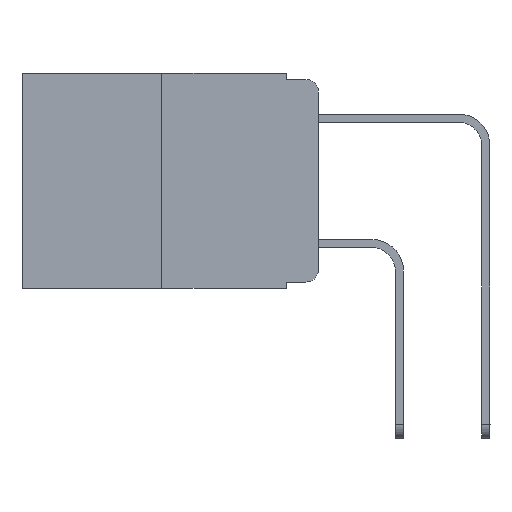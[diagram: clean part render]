
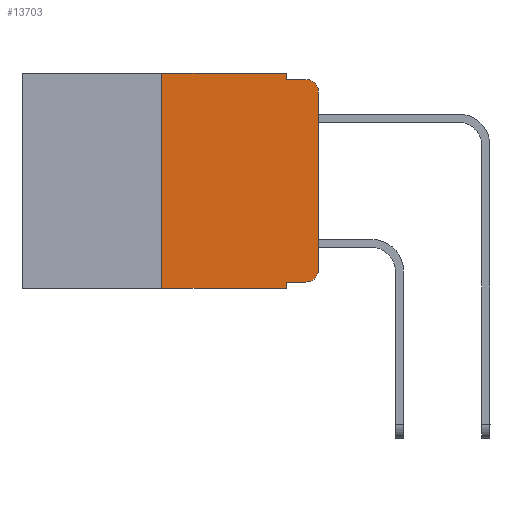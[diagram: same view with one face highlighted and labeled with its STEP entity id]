
A CAD part, left-side view. The second image highlights one B-rep face of the part: STEP entity #13703.
In plain terms, the highlighted planar face has unit normal (-1, 0, 0).
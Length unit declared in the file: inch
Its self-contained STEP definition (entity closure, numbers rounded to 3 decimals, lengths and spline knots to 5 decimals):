
#487 = DIRECTION ( 'NONE',  ( 0., -1., 0. ) ) ;
#741 = EDGE_CURVE ( 'NONE', #13259, #19435, #17257, .T. ) ;
#805 = DIRECTION ( 'NONE',  ( 0., -1., 0. ) ) ;
#1256 = CARTESIAN_POINT ( 'NONE',  ( 0., 0.02, -0.333 ) ) ;
#1263 = VERTEX_POINT ( 'NONE', #3067 ) ;
#1503 = LINE ( 'NONE', #21283, #15913 ) ;
#2000 = EDGE_CURVE ( 'NONE', #12940, #22669, #3964, .T. ) ;
#2510 = LINE ( 'NONE', #9604, #2660 ) ;
#2660 = VECTOR ( 'NONE', #16778, 39.37008 ) ;
#3067 = CARTESIAN_POINT ( 'NONE',  ( 0., 0.051, -0.333 ) ) ;
#3137 = LINE ( 'NONE', #13869, #8609 ) ;
#3624 = DIRECTION ( 'NONE',  ( 0., -1., 0. ) ) ;
#3964 = LINE ( 'NONE', #22002, #16583 ) ;
#4494 = VERTEX_POINT ( 'NONE', #10159 ) ;
#4611 = DIRECTION ( 'NONE',  ( 0., 0., 1. ) ) ;
#4775 = ORIENTED_EDGE ( 'NONE', *, *, #2000, .F. ) ;
#5005 = EDGE_LOOP ( 'NONE', ( #12325, #11528, #4775, #9613, #15126, #9640, #8739, #16223, #13482, #19015 ) ) ;
#5130 = CIRCLE ( 'NONE', #20851, 0.02 ) ;
#5294 = CARTESIAN_POINT ( 'NONE',  ( 0., 0.25, 0. ) ) ;
#5655 = VECTOR ( 'NONE', #4611, 39.37008 ) ;
#5818 = AXIS2_PLACEMENT_3D ( 'NONE', #16715, #21879, #11427 ) ;
#5894 = CARTESIAN_POINT ( 'NONE',  ( 0., 0.25, -0.343 ) ) ;
#6029 = CARTESIAN_POINT ( 'NONE',  ( 0., 0.02, -0.03 ) ) ;
#6677 = DIRECTION ( 'NONE',  ( 1., 0., 0. ) ) ;
#6683 = EDGE_CURVE ( 'NONE', #19435, #22669, #5130, .T. ) ;
#6791 = DIRECTION ( 'NONE',  ( 0., 0., -1. ) ) ;
#7473 = CARTESIAN_POINT ( 'NONE',  ( 0., 0., -0.03 ) ) ;
#8103 = CARTESIAN_POINT ( 'NONE',  ( 0., 0., 0. ) ) ;
#8246 = CARTESIAN_POINT ( 'NONE',  ( 0., 0.051, 0. ) ) ;
#8609 = VECTOR ( 'NONE', #19171, 39.37008 ) ;
#8739 = ORIENTED_EDGE ( 'NONE', *, *, #12901, .T. ) ;
#8962 = CARTESIAN_POINT ( 'NONE',  ( 0., 0.051, -0.01 ) ) ;
#9604 = CARTESIAN_POINT ( 'NONE',  ( 0., 0.051, 0. ) ) ;
#9613 = ORIENTED_EDGE ( 'NONE', *, *, #19042, .F. ) ;
#9640 = ORIENTED_EDGE ( 'NONE', *, *, #21232, .F. ) ;
#9706 = VECTOR ( 'NONE', #15413, 39.37008 ) ;
#9901 = CARTESIAN_POINT ( 'NONE',  ( 0., 0.473, 0. ) ) ;
#9912 = CIRCLE ( 'NONE', #5818, 0.02 ) ;
#10159 = CARTESIAN_POINT ( 'NONE',  ( 0., 0.051, 0. ) ) ;
#11427 = DIRECTION ( 'NONE',  ( 0., 0., -1. ) ) ;
#11528 = ORIENTED_EDGE ( 'NONE', *, *, #6683, .T. ) ;
#12189 = AXIS2_PLACEMENT_3D ( 'NONE', #14177, #6677, #6791 ) ;
#12325 = ORIENTED_EDGE ( 'NONE', *, *, #741, .T. ) ;
#12428 = FACE_OUTER_BOUND ( 'NONE', #5005, .T. ) ;
#12901 = EDGE_CURVE ( 'NONE', #13462, #17207, #1503, .T. ) ;
#12940 = VERTEX_POINT ( 'NONE', #8962 ) ;
#12971 = VECTOR ( 'NONE', #487, 39.37008 ) ;
#12981 = EDGE_CURVE ( 'NONE', #18723, #13259, #9912, .T. ) ;
#13259 = VERTEX_POINT ( 'NONE', #21485 ) ;
#13462 = VERTEX_POINT ( 'NONE', #5894 ) ;
#13482 = ORIENTED_EDGE ( 'NONE', *, *, #15523, .T. ) ;
#13703 = ADVANCED_FACE ( 'NONE', ( #12428 ), #17712, .F. ) ;
#13869 = CARTESIAN_POINT ( 'NONE',  ( 0., 0.25, 0. ) ) ;
#14177 = CARTESIAN_POINT ( 'NONE',  ( 0., 0.473, 0. ) ) ;
#15126 = ORIENTED_EDGE ( 'NONE', *, *, #20970, .F. ) ;
#15413 = DIRECTION ( 'NONE',  ( 0., 0., -1. ) ) ;
#15523 = EDGE_CURVE ( 'NONE', #1263, #18723, #18278, .T. ) ;
#15913 = VECTOR ( 'NONE', #16009, 39.37008 ) ;
#16009 = DIRECTION ( 'NONE',  ( 0., -1., 0. ) ) ;
#16223 = ORIENTED_EDGE ( 'NONE', *, *, #18736, .F. ) ;
#16583 = VECTOR ( 'NONE', #3624, 39.37008 ) ;
#16715 = CARTESIAN_POINT ( 'NONE',  ( 0., 0.02, -0.313 ) ) ;
#16778 = DIRECTION ( 'NONE',  ( 0., 0., -1. ) ) ;
#17207 = VERTEX_POINT ( 'NONE', #21731 ) ;
#17257 = LINE ( 'NONE', #8103, #5655 ) ;
#17511 = VERTEX_POINT ( 'NONE', #5294 ) ;
#17712 = PLANE ( 'NONE',  #12189 ) ;
#18159 = CARTESIAN_POINT ( 'NONE',  ( 0., 0.051, -0.333 ) ) ;
#18278 = LINE ( 'NONE', #18159, #12971 ) ;
#18592 = DIRECTION ( 'NONE',  ( -1., 0., 0. ) ) ;
#18723 = VERTEX_POINT ( 'NONE', #1256 ) ;
#18736 = EDGE_CURVE ( 'NONE', #1263, #17207, #22691, .T. ) ;
#19015 = ORIENTED_EDGE ( 'NONE', *, *, #12981, .T. ) ;
#19042 = EDGE_CURVE ( 'NONE', #4494, #12940, #2510, .T. ) ;
#19171 = DIRECTION ( 'NONE',  ( 0., 0., 1. ) ) ;
#19435 = VERTEX_POINT ( 'NONE', #7473 ) ;
#20332 = CARTESIAN_POINT ( 'NONE',  ( 0., 0.02, -0.01 ) ) ;
#20336 = DIRECTION ( 'NONE',  ( 0., 0., -1. ) ) ;
#20475 = LINE ( 'NONE', #9901, #21342 ) ;
#20851 = AXIS2_PLACEMENT_3D ( 'NONE', #6029, #18592, #20336 ) ;
#20970 = EDGE_CURVE ( 'NONE', #17511, #4494, #20475, .T. ) ;
#21232 = EDGE_CURVE ( 'NONE', #13462, #17511, #3137, .T. ) ;
#21283 = CARTESIAN_POINT ( 'NONE',  ( 0., 0.473, -0.343 ) ) ;
#21342 = VECTOR ( 'NONE', #805, 39.37008 ) ;
#21485 = CARTESIAN_POINT ( 'NONE',  ( 0., 0., -0.313 ) ) ;
#21731 = CARTESIAN_POINT ( 'NONE',  ( 0., 0.051, -0.343 ) ) ;
#21879 = DIRECTION ( 'NONE',  ( -1., 0., 0. ) ) ;
#22002 = CARTESIAN_POINT ( 'NONE',  ( 0., 0.051, -0.01 ) ) ;
#22669 = VERTEX_POINT ( 'NONE', #20332 ) ;
#22691 = LINE ( 'NONE', #8246, #9706 ) ;
